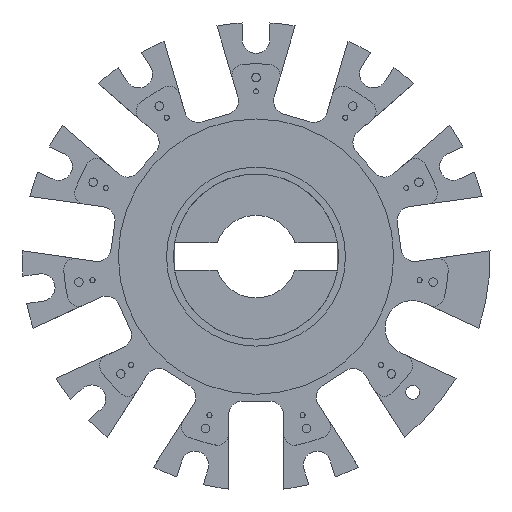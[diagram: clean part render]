
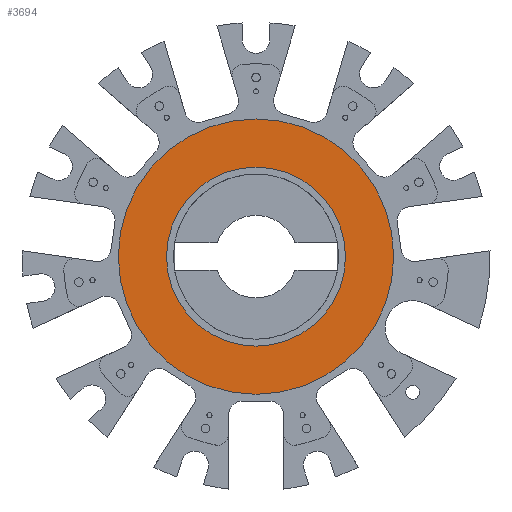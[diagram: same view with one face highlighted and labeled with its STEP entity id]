
A CAD part, front view. The second image highlights one B-rep face of the part: STEP entity #3694.
In plain terms, the highlighted planar face has unit normal (0, -1, 0).
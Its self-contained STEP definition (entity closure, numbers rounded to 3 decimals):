
#261 = EDGE_LOOP ( 'NONE', ( #6242, #2697 ) ) ;
#526 = ORIENTED_EDGE ( 'NONE', *, *, #2167, .F. ) ;
#527 = CIRCLE ( 'NONE', #2120, 50. ) ;
#557 = VERTEX_POINT ( 'NONE', #2729 ) ;
#630 = CARTESIAN_POINT ( 'NONE',  ( 0., 27.5, -32.5 ) ) ;
#998 = FACE_OUTER_BOUND ( 'NONE', #261, .T. ) ;
#1083 = ORIENTED_EDGE ( 'NONE', *, *, #5734, .F. ) ;
#1566 = AXIS2_PLACEMENT_3D ( 'NONE', #1650, #7206, #7096 ) ;
#1592 = CARTESIAN_POINT ( 'NONE',  ( 0., 27.5, -50. ) ) ;
#1650 = CARTESIAN_POINT ( 'NONE',  ( 0., 27.5, 0. ) ) ;
#1654 = CIRCLE ( 'NONE', #4001, 32.5 ) ;
#1765 = CARTESIAN_POINT ( 'NONE',  ( 0., 27.5, 0. ) ) ;
#1900 = DIRECTION ( 'NONE',  ( 0., -1., 0. ) ) ;
#2120 = AXIS2_PLACEMENT_3D ( 'NONE', #4745, #2262, #4640 ) ;
#2167 = EDGE_CURVE ( 'NONE', #3752, #4300, #1654, .T. ) ;
#2262 = DIRECTION ( 'NONE',  ( 0., -1., 0. ) ) ;
#2266 = CARTESIAN_POINT ( 'NONE',  ( 0., 27.5, 0. ) ) ;
#2357 = DIRECTION ( 'NONE',  ( 0., -1., 0. ) ) ;
#2697 = ORIENTED_EDGE ( 'NONE', *, *, #6058, .T. ) ;
#2729 = CARTESIAN_POINT ( 'NONE',  ( 0., 27.5, 50. ) ) ;
#2733 = CARTESIAN_POINT ( 'NONE',  ( 0., 27.5, 32.5 ) ) ;
#2864 = EDGE_LOOP ( 'NONE', ( #1083, #526 ) ) ;
#2885 = DIRECTION ( 'NONE',  ( 0., -1., 0. ) ) ;
#3449 = AXIS2_PLACEMENT_3D ( 'NONE', #5109, #1900, #6240 ) ;
#3694 = ADVANCED_FACE ( 'NONE', ( #3891, #998 ), #5715, .T. ) ;
#3752 = VERTEX_POINT ( 'NONE', #2733 ) ;
#3891 = FACE_BOUND ( 'NONE', #2864, .T. ) ;
#4001 = AXIS2_PLACEMENT_3D ( 'NONE', #2266, #2885, #6634 ) ;
#4300 = VERTEX_POINT ( 'NONE', #630 ) ;
#4640 = DIRECTION ( 'NONE',  ( 0., 0., -1. ) ) ;
#4745 = CARTESIAN_POINT ( 'NONE',  ( 0., 27.5, 0. ) ) ;
#5109 = CARTESIAN_POINT ( 'NONE',  ( 0., 27.5, 0. ) ) ;
#5715 = PLANE ( 'NONE',  #3449 ) ;
#5734 = EDGE_CURVE ( 'NONE', #4300, #3752, #7937, .T. ) ;
#6021 = EDGE_CURVE ( 'NONE', #7278, #557, #527, .T. ) ;
#6058 = EDGE_CURVE ( 'NONE', #557, #7278, #7468, .T. ) ;
#6240 = DIRECTION ( 'NONE',  ( 0., 0., -1. ) ) ;
#6242 = ORIENTED_EDGE ( 'NONE', *, *, #6021, .T. ) ;
#6634 = DIRECTION ( 'NONE',  ( 0., 0., -1. ) ) ;
#6776 = AXIS2_PLACEMENT_3D ( 'NONE', #1765, #2357, #7295 ) ;
#7096 = DIRECTION ( 'NONE',  ( 0., 0., -1. ) ) ;
#7206 = DIRECTION ( 'NONE',  ( 0., -1., 0. ) ) ;
#7278 = VERTEX_POINT ( 'NONE', #1592 ) ;
#7295 = DIRECTION ( 'NONE',  ( 0., 0., -1. ) ) ;
#7468 = CIRCLE ( 'NONE', #1566, 50. ) ;
#7937 = CIRCLE ( 'NONE', #6776, 32.5 ) ;
